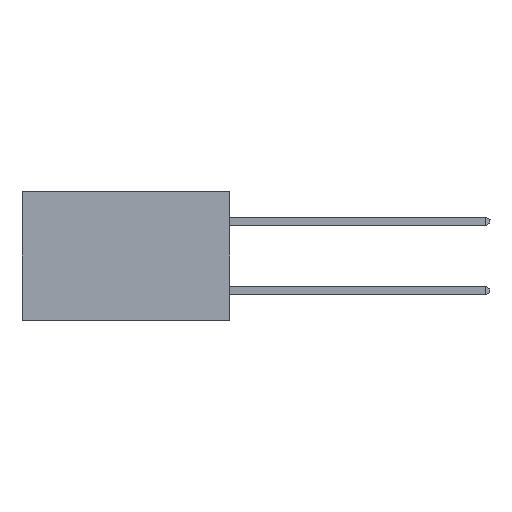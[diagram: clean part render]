
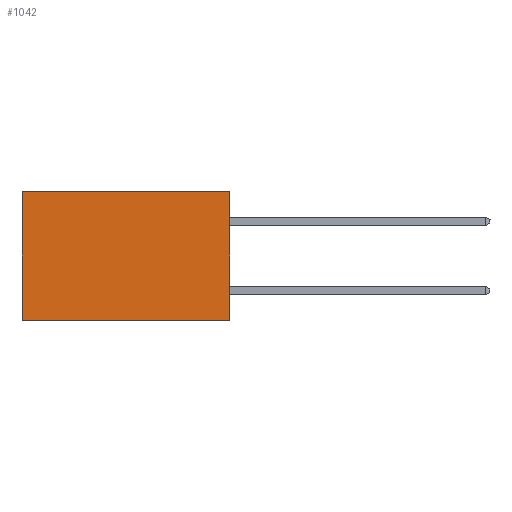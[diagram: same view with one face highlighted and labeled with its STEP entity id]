
A CAD part, left-side view. The second image highlights one B-rep face of the part: STEP entity #1042.
In plain terms, the highlighted planar face has unit normal (-1, 0, 0).
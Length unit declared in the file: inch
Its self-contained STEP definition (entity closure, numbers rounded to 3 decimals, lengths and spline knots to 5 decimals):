
#200 = DIRECTION ( 'NONE',  ( 0., 0., -1. ) ) ;
#875 = ORIENTED_EDGE ( 'NONE', *, *, #17087, .F. ) ;
#1006 = LINE ( 'NONE', #14353, #10905 ) ;
#1042 = ADVANCED_FACE ( 'NONE', ( #16094 ), #15145, .F. ) ;
#2248 = CARTESIAN_POINT ( 'NONE',  ( 0.298, 0.6, 0. ) ) ;
#2467 = DIRECTION ( 'NONE',  ( 0., 1., 0. ) ) ;
#3090 = LINE ( 'NONE', #14146, #17030 ) ;
#3237 = EDGE_CURVE ( 'NONE', #12689, #6634, #9920, .T. ) ;
#3255 = ORIENTED_EDGE ( 'NONE', *, *, #11742, .T. ) ;
#3506 = VERTEX_POINT ( 'NONE', #2248 ) ;
#3543 = CARTESIAN_POINT ( 'NONE',  ( 0.298, 0., 0. ) ) ;
#4052 = CARTESIAN_POINT ( 'NONE',  ( 0.298, 0., -0.37 ) ) ;
#5121 = EDGE_CURVE ( 'NONE', #3506, #14911, #3090, .T. ) ;
#5680 = CARTESIAN_POINT ( 'NONE',  ( 0.298, 0., 0. ) ) ;
#5849 = DIRECTION ( 'NONE',  ( 1., 0., 0. ) ) ;
#6620 = CARTESIAN_POINT ( 'NONE',  ( 0.298, 0.6, -0.37 ) ) ;
#6634 = VERTEX_POINT ( 'NONE', #4052 ) ;
#7047 = DIRECTION ( 'NONE',  ( 0., 0., -1. ) ) ;
#8298 = AXIS2_PLACEMENT_3D ( 'NONE', #5680, #5849, #7047 ) ;
#8704 = ORIENTED_EDGE ( 'NONE', *, *, #5121, .T. ) ;
#8837 = CARTESIAN_POINT ( 'NONE',  ( 0.298, 0., 0. ) ) ;
#9920 = LINE ( 'NONE', #8837, #15815 ) ;
#10366 = CARTESIAN_POINT ( 'NONE',  ( 0.298, 0., 0. ) ) ;
#10905 = VECTOR ( 'NONE', #2467, 39.37008 ) ;
#11690 = DIRECTION ( 'NONE',  ( 0., 1., 0. ) ) ;
#11742 = EDGE_CURVE ( 'NONE', #12689, #3506, #12559, .T. ) ;
#12151 = ORIENTED_EDGE ( 'NONE', *, *, #3237, .F. ) ;
#12160 = EDGE_LOOP ( 'NONE', ( #8704, #875, #12151, #3255 ) ) ;
#12559 = LINE ( 'NONE', #10366, #16849 ) ;
#12689 = VERTEX_POINT ( 'NONE', #3543 ) ;
#14146 = CARTESIAN_POINT ( 'NONE',  ( 0.298, 0.6, 0. ) ) ;
#14353 = CARTESIAN_POINT ( 'NONE',  ( 0.298, 0., -0.37 ) ) ;
#14911 = VERTEX_POINT ( 'NONE', #6620 ) ;
#15145 = PLANE ( 'NONE',  #8298 ) ;
#15815 = VECTOR ( 'NONE', #16987, 39.37008 ) ;
#16094 = FACE_OUTER_BOUND ( 'NONE', #12160, .T. ) ;
#16849 = VECTOR ( 'NONE', #11690, 39.37008 ) ;
#16987 = DIRECTION ( 'NONE',  ( 0., 0., -1. ) ) ;
#17030 = VECTOR ( 'NONE', #200, 39.37008 ) ;
#17087 = EDGE_CURVE ( 'NONE', #6634, #14911, #1006, .T. ) ;
